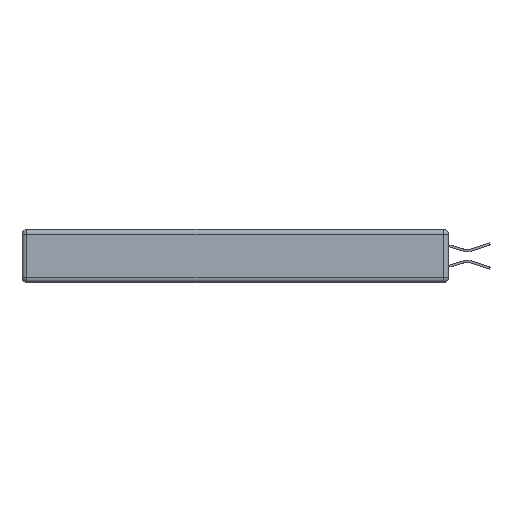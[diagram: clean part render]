
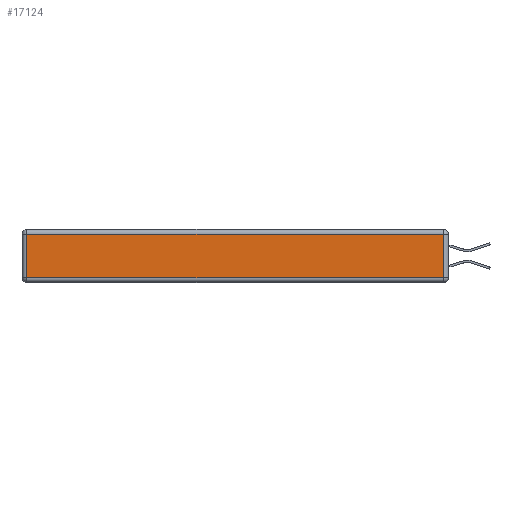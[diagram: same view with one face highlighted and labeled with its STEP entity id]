
A CAD part, left-side view. The second image highlights one B-rep face of the part: STEP entity #17124.
In plain terms, the highlighted planar face has unit normal (-1, 0, 0).
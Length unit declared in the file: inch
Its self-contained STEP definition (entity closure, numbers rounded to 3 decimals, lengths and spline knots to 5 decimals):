
#220 = VECTOR ( 'NONE', #7235, 39.37008 ) ;
#875 = VERTEX_POINT ( 'NONE', #14512 ) ;
#1020 = CARTESIAN_POINT ( 'NONE',  ( 0., 2.72, -0.03 ) ) ;
#1923 = EDGE_CURVE ( 'NONE', #875, #13721, #13157, .T. ) ;
#2417 = FACE_OUTER_BOUND ( 'NONE', #17908, .T. ) ;
#2994 = EDGE_CURVE ( 'NONE', #13721, #10327, #17733, .T. ) ;
#3543 = ORIENTED_EDGE ( 'NONE', *, *, #7635, .T. ) ;
#4231 = DIRECTION ( 'NONE',  ( 0., -1., 0. ) ) ;
#5992 = PLANE ( 'NONE',  #17493 ) ;
#6017 = CARTESIAN_POINT ( 'NONE',  ( 0., 0.03, -0.03 ) ) ;
#6256 = LINE ( 'NONE', #9797, #15269 ) ;
#6394 = CARTESIAN_POINT ( 'NONE',  ( 0., 2.72, -0.313 ) ) ;
#6441 = DIRECTION ( 'NONE',  ( 0., 0., -1. ) ) ;
#7235 = DIRECTION ( 'NONE',  ( 0., 1., 0. ) ) ;
#7635 = EDGE_CURVE ( 'NONE', #15099, #875, #6256, .T. ) ;
#8664 = EDGE_CURVE ( 'NONE', #10327, #15099, #15233, .T. ) ;
#9358 = DIRECTION ( 'NONE',  ( 0., 0., 1. ) ) ;
#9797 = CARTESIAN_POINT ( 'NONE',  ( 0., 0., -0.313 ) ) ;
#10289 = CARTESIAN_POINT ( 'NONE',  ( 0., 0., -0.343 ) ) ;
#10327 = VERTEX_POINT ( 'NONE', #1020 ) ;
#11115 = CARTESIAN_POINT ( 'NONE',  ( 0., 0.03, -0.343 ) ) ;
#11503 = VECTOR ( 'NONE', #6441, 39.37008 ) ;
#11845 = VECTOR ( 'NONE', #15414, 39.37008 ) ;
#12640 = CARTESIAN_POINT ( 'NONE',  ( 0., 2.75, -0.03 ) ) ;
#12718 = ORIENTED_EDGE ( 'NONE', *, *, #8664, .T. ) ;
#13083 = DIRECTION ( 'NONE',  ( -1., 0., 0. ) ) ;
#13157 = LINE ( 'NONE', #11115, #11845 ) ;
#13721 = VERTEX_POINT ( 'NONE', #6017 ) ;
#14512 = CARTESIAN_POINT ( 'NONE',  ( 0., 0.03, -0.313 ) ) ;
#15099 = VERTEX_POINT ( 'NONE', #6394 ) ;
#15113 = ORIENTED_EDGE ( 'NONE', *, *, #1923, .T. ) ;
#15233 = LINE ( 'NONE', #16081, #11503 ) ;
#15269 = VECTOR ( 'NONE', #4231, 39.37008 ) ;
#15414 = DIRECTION ( 'NONE',  ( 0., 0., 1. ) ) ;
#16081 = CARTESIAN_POINT ( 'NONE',  ( 0., 2.72, -0.343 ) ) ;
#16154 = ORIENTED_EDGE ( 'NONE', *, *, #2994, .T. ) ;
#17124 = ADVANCED_FACE ( 'NONE', ( #2417 ), #5992, .T. ) ;
#17493 = AXIS2_PLACEMENT_3D ( 'NONE', #10289, #13083, #9358 ) ;
#17733 = LINE ( 'NONE', #12640, #220 ) ;
#17908 = EDGE_LOOP ( 'NONE', ( #3543, #15113, #16154, #12718 ) ) ;
